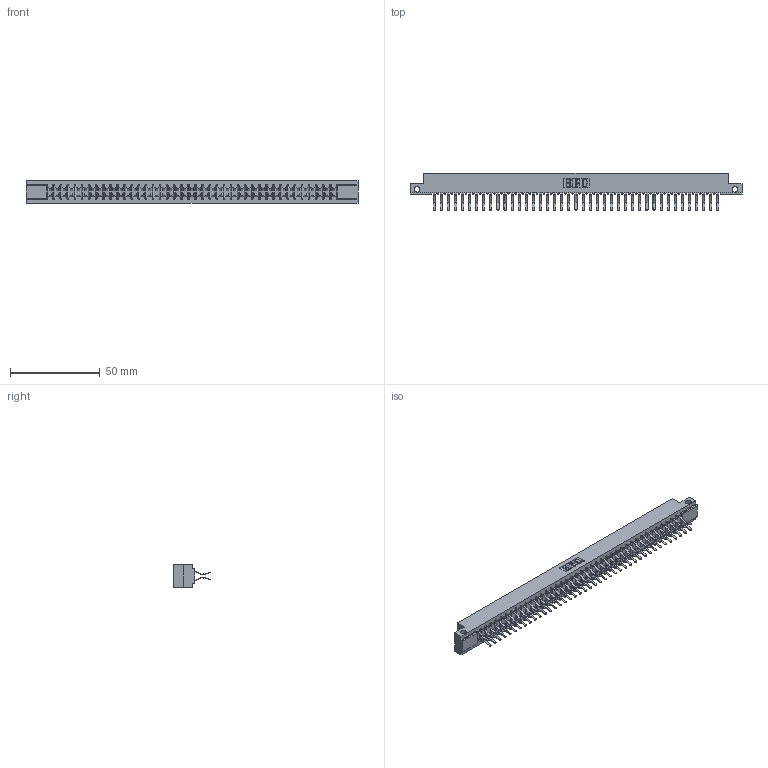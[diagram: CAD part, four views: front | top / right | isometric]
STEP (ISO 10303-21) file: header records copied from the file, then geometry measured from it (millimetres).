
FILE_DESCRIPTION (( 'STEP AP203' ), '1' );
FILE_NAME ('357-082-460-212.STEP', '2020-10-04T08:57:45', ( '' ), ( '' ), 'SwSTEP 2.0', 'SolidWorks 2020', '' );
FILE_SCHEMA (( 'CONFIG_CONTROL_DESIGN' ));
Length unit declared in the file: inch
Products named in the file (3): 307 Part_.128 Dia Side Mounting Holes; 307-290-001_560; 357-082-460-212
Assembly tree (83 placements, depth 2):
  357-082-460-212
    307 Part_.128 Dia Side Mounting Holes
    307-290-001_560  x82
Bounding box: 185.47 x 20.73 x 12.7 mm (x, y, z)
Volume: 19675.6 mm3; surface area: 24589.9 mm2
Topology: 83 solids, 83 shells, 4260 faces, 11967 edges, 7754 vertices
Faces by surface type: plane 2776, cylinder 1400, sphere 84
Entity records: 36690 total; most frequent: CARTESIAN_POINT 6001, ORIENTED_EDGE 5946, DIRECTION 5879, EDGE_CURVE 2973, LINE 2279, VECTOR 2279, VERTEX_POINT 1922, AXIS2_PLACEMENT_3D 1800
